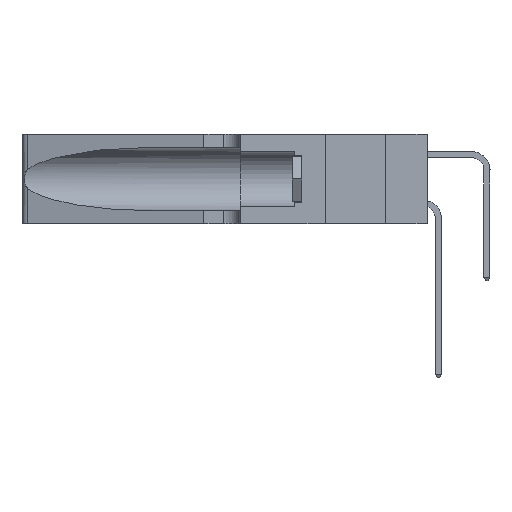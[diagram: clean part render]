
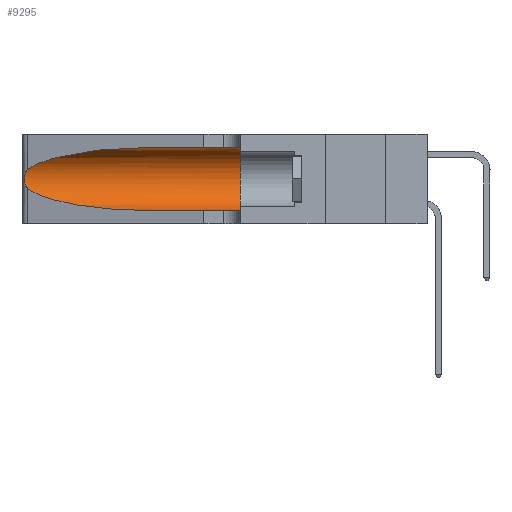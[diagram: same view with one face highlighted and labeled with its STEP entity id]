
A CAD part, left-side view. The second image highlights one B-rep face of the part: STEP entity #9295.
In plain terms, the highlighted cylindrical face has radius 3.308 mm (diameter 6.617 mm), a partial arc.
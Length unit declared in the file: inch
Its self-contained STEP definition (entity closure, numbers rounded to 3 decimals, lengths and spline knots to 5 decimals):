
#180 = VECTOR ( 'NONE', #12763, 39.37008 ) ;
#317 = B_SPLINE_CURVE_WITH_KNOTS ( 'NONE', 3,
 ( #8833, #3573, #18968, #11415, #28982, #13972, #31502, #16530, #1001, #19077, #3691, #21591, #6326, #24101 ),
 .UNSPECIFIED., .F., .F.,
 ( 4, 2, 2, 2, 2, 2, 4 ),
 ( 0., 0.00027, 0.00053, 0.00107, 0.0016, 0.00187, 0.00214 ),
 .UNSPECIFIED. ) ;
#443 = ORIENTED_EDGE ( 'NONE', *, *, #32979, .T. ) ;
#1001 = CARTESIAN_POINT ( 'NONE',  ( 0.26017, 1.23833, 0.17102 ) ) ;
#1574 = CARTESIAN_POINT ( 'NONE',  ( 0.18966, 0.96281, 0.31525 ) ) ;
#3008 = EDGE_CURVE ( 'NONE', #7696, #5147, #317, .T. ) ;
#3573 = CARTESIAN_POINT ( 'NONE',  ( 0.25555, 1.22994, 0.2215 ) ) ;
#3683 = CARTESIAN_POINT ( 'NONE',  ( 0.1305, 1.61858, 0.185 ) ) ;
#3691 = CARTESIAN_POINT ( 'NONE',  ( 0.25789, 1.23486, 0.15765 ) ) ;
#4969 = VERTEX_POINT ( 'NONE', #26198 ) ;
#5106 = CARTESIAN_POINT ( 'NONE',  ( 0.18966, 0.96281, 0.05475 ) ) ;
#5147 = VERTEX_POINT ( 'NONE', #6698 ) ;
#5424 = EDGE_CURVE ( 'NONE', #5147, #9426, #22974, .T. ) ;
#6326 = CARTESIAN_POINT ( 'NONE',  ( 0.25555, 1.22993, 0.14849 ) ) ;
#6698 = CARTESIAN_POINT ( 'NONE',  ( 0.25487, 1.22718, 0.14631 ) ) ;
#6972 = ORIENTED_EDGE ( 'NONE', *, *, #20032, .F. ) ;
#7204 = VERTEX_POINT ( 'NONE', #12109 ) ;
#7255 = CYLINDRICAL_SURFACE ( 'NONE', #25862, 0.13025 ) ;
#7696 = VERTEX_POINT ( 'NONE', #31612 ) ;
#8545 = CARTESIAN_POINT ( 'NONE',  ( 0.1305, 0.35, 0.31525 ) ) ;
#8619 = DIRECTION ( 'NONE',  ( 0., 1., 0. ) ) ;
#8833 = CARTESIAN_POINT ( 'NONE',  ( 0.25487, 1.22718, 0.22369 ) ) ;
#9218 = EDGE_LOOP ( 'NONE', ( #443, #26131, #16229, #12106, #6972, #15613 ) ) ;
#9295 = ADVANCED_FACE ( 'NONE', ( #27403 ), #7255, .F. ) ;
#9426 = VERTEX_POINT ( 'NONE', #11938 ) ;
#9650 = EDGE_CURVE ( 'NONE', #4969, #17837, #10477, .T. ) ;
#9654 = VECTOR ( 'NONE', #17919, 39.37008 ) ;
#10477 = LINE ( 'NONE', #15399, #9654 ) ;
#11415 = CARTESIAN_POINT ( 'NONE',  ( 0.25787, 1.23484, 0.2124 ) ) ;
#11938 = CARTESIAN_POINT ( 'NONE',  ( 0.1305, 0.72297, 0.05475 ) ) ;
#12028 = CARTESIAN_POINT ( 'NONE',  ( 0.2373, 1.15595, 0.28018 ) ) ;
#12106 = ORIENTED_EDGE ( 'NONE', *, *, #28161, .T. ) ;
#12109 = CARTESIAN_POINT ( 'NONE',  ( 0.1305, 0.35, 0.05475 ) ) ;
#12763 = DIRECTION ( 'NONE',  ( 0., -1., 0. ) ) ;
#13972 = CARTESIAN_POINT ( 'NONE',  ( 0.26018, 1.23835, 0.19895 ) ) ;
#15399 = CARTESIAN_POINT ( 'NONE',  ( 0.1305, 1.61858, 0.31525 ) ) ;
#15613 = ORIENTED_EDGE ( 'NONE', *, *, #9650, .F. ) ;
#16229 = ORIENTED_EDGE ( 'NONE', *, *, #5424, .T. ) ;
#16530 = CARTESIAN_POINT ( 'NONE',  ( 0.26075, 1.23896, 0.178 ) ) ;
#17837 = VERTEX_POINT ( 'NONE', #8545 ) ;
#17866 = CARTESIAN_POINT ( 'NONE',  ( 0.25487, 1.22718, 0.14631 ) ) ;
#17919 = DIRECTION ( 'NONE',  ( 0., -1., 0. ) ) ;
#18968 = CARTESIAN_POINT ( 'NONE',  ( 0.25639, 1.23184, 0.21858 ) ) ;
#19077 = CARTESIAN_POINT ( 'NONE',  ( 0.25856, 1.23593, 0.16098 ) ) ;
#19168 = AXIS2_PLACEMENT_3D ( 'NONE', #23790, #8619, #26282 ) ;
#19585 = CARTESIAN_POINT ( 'NONE',  ( 0.1305, 0.72297, 0.31525 ) ) ;
#20032 = EDGE_CURVE ( 'NONE', #17837, #7204, #24733, .T. ) ;
#20414 = CARTESIAN_POINT ( 'NONE',  ( 0.2373, 1.15595, 0.08982 ) ) ;
#21583 = DIRECTION ( 'NONE',  ( 0., -1., 0. ) ) ;
#21591 = CARTESIAN_POINT ( 'NONE',  ( 0.25639, 1.23186, 0.15144 ) ) ;
#22920 = CARTESIAN_POINT ( 'NONE',  ( 0.1305, 0.72297, 0.05475 ) ) ;
#22974 =( BOUNDED_CURVE ( )  B_SPLINE_CURVE ( 3, ( #17866, #20414, #5106, #22920 ),
 .UNSPECIFIED., .F., .F. ) 
 B_SPLINE_CURVE_WITH_KNOTS ( ( 4, 4 ),
 ( 3.44316, 4.71239 ),
 .UNSPECIFIED. ) 
 CURVE ( )  GEOMETRIC_REPRESENTATION_ITEM ( )  RATIONAL_B_SPLINE_CURVE ( ( 1., 0.87, 0.87, 1. ) ) 
 REPRESENTATION_ITEM ( '' )  );
#23790 = CARTESIAN_POINT ( 'NONE',  ( 0.1305, 0.35, 0.185 ) ) ;
#24101 = CARTESIAN_POINT ( 'NONE',  ( 0.25487, 1.22718, 0.14631 ) ) ;
#24733 = CIRCLE ( 'NONE', #19168, 0.13025 ) ;
#25862 = AXIS2_PLACEMENT_3D ( 'NONE', #3683, #21583, #26482 ) ;
#26131 = ORIENTED_EDGE ( 'NONE', *, *, #3008, .T. ) ;
#26198 = CARTESIAN_POINT ( 'NONE',  ( 0.1305, 0.72297, 0.31525 ) ) ;
#26282 = DIRECTION ( 'NONE',  ( 0., 0., 1. ) ) ;
#26482 = DIRECTION ( 'NONE',  ( 0., 0., -1. ) ) ;
#27333 =( BOUNDED_CURVE ( )  B_SPLINE_CURVE ( 3, ( #19585, #1574, #12028, #29590 ),
 .UNSPECIFIED., .F., .F. ) 
 B_SPLINE_CURVE_WITH_KNOTS ( ( 4, 4 ),
 ( 1.5708, 2.84003 ),
 .UNSPECIFIED. ) 
 CURVE ( )  GEOMETRIC_REPRESENTATION_ITEM ( )  RATIONAL_B_SPLINE_CURVE ( ( 1., 0.87, 0.87, 1. ) ) 
 REPRESENTATION_ITEM ( '' )  );
#27383 = LINE ( 'NONE', #30288, #180 ) ;
#27403 = FACE_OUTER_BOUND ( 'NONE', #9218, .T. ) ;
#28161 = EDGE_CURVE ( 'NONE', #9426, #7204, #27383, .T. ) ;
#28982 = CARTESIAN_POINT ( 'NONE',  ( 0.25854, 1.2359, 0.20912 ) ) ;
#29590 = CARTESIAN_POINT ( 'NONE',  ( 0.25487, 1.22718, 0.22369 ) ) ;
#30288 = CARTESIAN_POINT ( 'NONE',  ( 0.1305, 1.61858, 0.05475 ) ) ;
#31502 = CARTESIAN_POINT ( 'NONE',  ( 0.26075, 1.23896, 0.19203 ) ) ;
#31612 = CARTESIAN_POINT ( 'NONE',  ( 0.25487, 1.22718, 0.22369 ) ) ;
#32979 = EDGE_CURVE ( 'NONE', #4969, #7696, #27333, .T. ) ;
